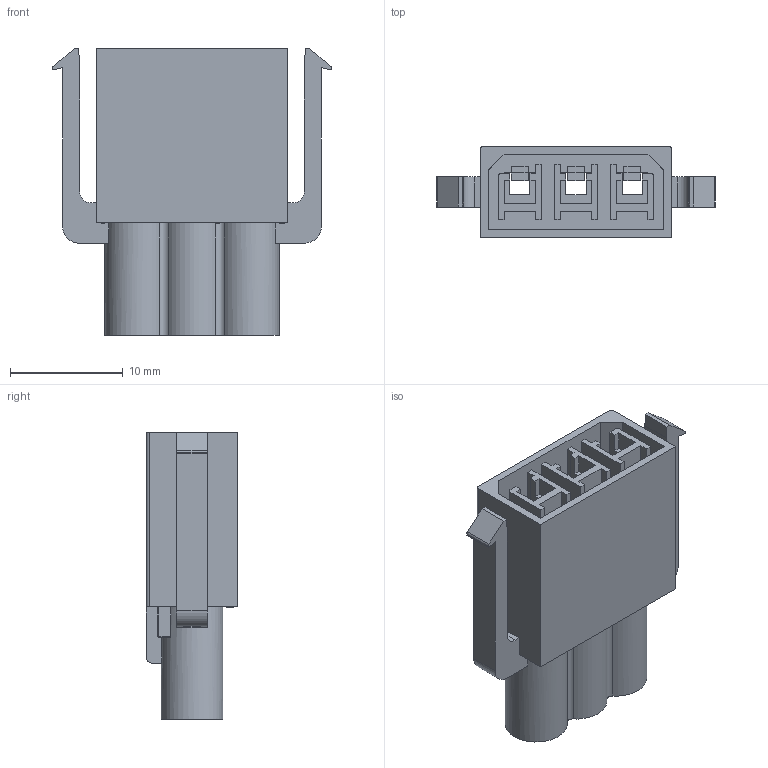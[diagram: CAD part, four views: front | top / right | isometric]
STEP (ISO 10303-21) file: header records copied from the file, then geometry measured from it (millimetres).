
FILE_DESCRIPTION (( 'STEP AP214' ), '1' );
FILE_NAME ('567-003-000-410.STEP', '2020-07-27T20:03:38', ( '' ), ( '' ), 'SwSTEP 2.0', 'SolidWorks 2020', '' );
FILE_SCHEMA (( 'AUTOMOTIVE_DESIGN' ));
Length unit declared in the file: millimetre
Products named in the file (1): 567-003-000-410
Bounding box: 24.8 x 8.1 x 25.5 mm (x, y, z)
Volume: 1389.7 mm3; surface area: 4028.3 mm2
Topology: 1 solids, 1 shells, 266 faces, 770 edges, 508 vertices
Faces by surface type: plane 209, cylinder 35, bspline 20, sphere 2
Entity records: 9698 total; most frequent: CARTESIAN_POINT 2773, ORIENTED_EDGE 1536, DIRECTION 1286, EDGE_CURVE 768, LINE 624, VECTOR 624, VERTEX_POINT 508, AXIS2_PLACEMENT_3D 331
